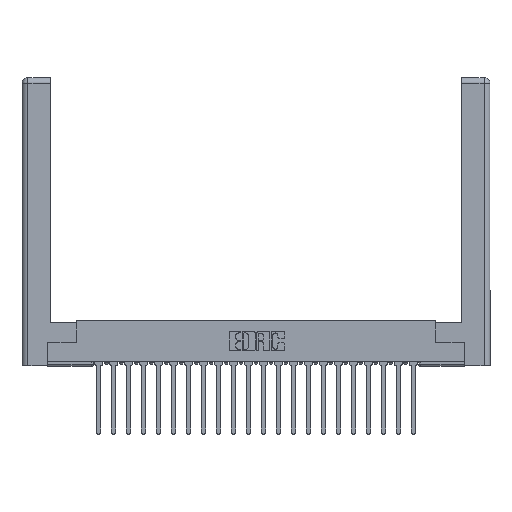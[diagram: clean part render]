
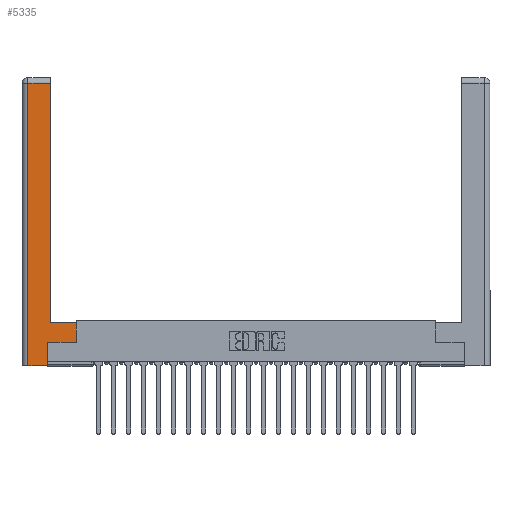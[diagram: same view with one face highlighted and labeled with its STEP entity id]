
A CAD part, top view. The second image highlights one B-rep face of the part: STEP entity #5335.
In plain terms, the highlighted planar face has unit normal (0, 0, 1).
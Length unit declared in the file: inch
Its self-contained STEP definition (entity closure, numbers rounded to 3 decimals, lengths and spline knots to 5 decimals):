
#131 = CARTESIAN_POINT ( 'NONE',  ( 0.0615, 2.94, 0. ) ) ;
#763 = VECTOR ( 'NONE', #1861, 39.37008 ) ;
#911 = EDGE_CURVE ( 'NONE', #6906, #17851, #3700, .T. ) ;
#1861 = DIRECTION ( 'NONE',  ( 0., 1., 0. ) ) ;
#2211 = DIRECTION ( 'NONE',  ( -1., 0., 0. ) ) ;
#2676 = VECTOR ( 'NONE', #22373, 39.37008 ) ;
#2912 = VECTOR ( 'NONE', #20176, 39.37008 ) ;
#2974 = LINE ( 'NONE', #18294, #2912 ) ;
#3685 = EDGE_CURVE ( 'NONE', #16562, #9395, #9204, .T. ) ;
#3700 = LINE ( 'NONE', #23017, #13595 ) ;
#4111 = LINE ( 'NONE', #131, #18956 ) ;
#4212 = FACE_OUTER_BOUND ( 'NONE', #11260, .T. ) ;
#4555 = LINE ( 'NONE', #8407, #15140 ) ;
#4575 = VERTEX_POINT ( 'NONE', #18118 ) ;
#4806 = CARTESIAN_POINT ( 'NONE',  ( 0.565, 0.45, 0. ) ) ;
#5335 = ADVANCED_FACE ( 'NONE', ( #4212 ), #17548, .F. ) ;
#5801 = DIRECTION ( 'NONE',  ( 0., 1., 0. ) ) ;
#5974 = EDGE_CURVE ( 'NONE', #4575, #16562, #4555, .T. ) ;
#6198 = CARTESIAN_POINT ( 'NONE',  ( 0., 0., 0. ) ) ;
#6542 = DIRECTION ( 'NONE',  ( 0., -1., 0. ) ) ;
#6906 = VERTEX_POINT ( 'NONE', #24538 ) ;
#7162 = ORIENTED_EDGE ( 'NONE', *, *, #12936, .T. ) ;
#7429 = LINE ( 'NONE', #13552, #24229 ) ;
#7552 = AXIS2_PLACEMENT_3D ( 'NONE', #6198, #19545, #23422 ) ;
#8185 = VERTEX_POINT ( 'NONE', #14827 ) ;
#8275 = VECTOR ( 'NONE', #14929, 39.37008 ) ;
#8407 = CARTESIAN_POINT ( 'NONE',  ( 0.0615, 0., 0. ) ) ;
#9204 = LINE ( 'NONE', #15975, #8275 ) ;
#9395 = VERTEX_POINT ( 'NONE', #11569 ) ;
#9710 = ORIENTED_EDGE ( 'NONE', *, *, #14147, .T. ) ;
#10265 = LINE ( 'NONE', #23746, #2676 ) ;
#11260 = EDGE_LOOP ( 'NONE', ( #15398, #7162, #13005, #13770, #14939, #9710, #16531, #13650 ) ) ;
#11569 = CARTESIAN_POINT ( 'NONE',  ( 0.265, 0., 0. ) ) ;
#12936 = EDGE_CURVE ( 'NONE', #8185, #4575, #4111, .T. ) ;
#13005 = ORIENTED_EDGE ( 'NONE', *, *, #5974, .T. ) ;
#13552 = CARTESIAN_POINT ( 'NONE',  ( 0.295, 0.45, 0. ) ) ;
#13595 = VECTOR ( 'NONE', #5801, 39.37008 ) ;
#13650 = ORIENTED_EDGE ( 'NONE', *, *, #23297, .T. ) ;
#13770 = ORIENTED_EDGE ( 'NONE', *, *, #3685, .T. ) ;
#14147 = EDGE_CURVE ( 'NONE', #21515, #6906, #10265, .T. ) ;
#14827 = CARTESIAN_POINT ( 'NONE',  ( 0.295, 2.94, 0. ) ) ;
#14929 = DIRECTION ( 'NONE',  ( 1., 0., 0. ) ) ;
#14936 = CARTESIAN_POINT ( 'NONE',  ( 0.0615, 0., 0. ) ) ;
#14939 = ORIENTED_EDGE ( 'NONE', *, *, #15290, .T. ) ;
#15050 = LINE ( 'NONE', #20807, #763 ) ;
#15140 = VECTOR ( 'NONE', #6542, 39.37008 ) ;
#15290 = EDGE_CURVE ( 'NONE', #9395, #21515, #15050, .T. ) ;
#15398 = ORIENTED_EDGE ( 'NONE', *, *, #20545, .T. ) ;
#15975 = CARTESIAN_POINT ( 'NONE',  ( 0.265, 0., 0. ) ) ;
#16531 = ORIENTED_EDGE ( 'NONE', *, *, #911, .T. ) ;
#16562 = VERTEX_POINT ( 'NONE', #14936 ) ;
#17548 = PLANE ( 'NONE',  #7552 ) ;
#17851 = VERTEX_POINT ( 'NONE', #4806 ) ;
#18118 = CARTESIAN_POINT ( 'NONE',  ( 0.0615, 2.94, 0. ) ) ;
#18294 = CARTESIAN_POINT ( 'NONE',  ( 0.295, 3., 0. ) ) ;
#18329 = CARTESIAN_POINT ( 'NONE',  ( 0.265, 0.245, 0. ) ) ;
#18637 = VERTEX_POINT ( 'NONE', #19205 ) ;
#18956 = VECTOR ( 'NONE', #19056, 39.37008 ) ;
#19056 = DIRECTION ( 'NONE',  ( -1., 0., 0. ) ) ;
#19205 = CARTESIAN_POINT ( 'NONE',  ( 0.295, 0.45, 0. ) ) ;
#19545 = DIRECTION ( 'NONE',  ( 0., 0., -1. ) ) ;
#20176 = DIRECTION ( 'NONE',  ( 0., 1., 0. ) ) ;
#20545 = EDGE_CURVE ( 'NONE', #18637, #8185, #2974, .T. ) ;
#20807 = CARTESIAN_POINT ( 'NONE',  ( 0.265, 0.245, 0. ) ) ;
#21515 = VERTEX_POINT ( 'NONE', #18329 ) ;
#22373 = DIRECTION ( 'NONE',  ( 1., 0., 0. ) ) ;
#23017 = CARTESIAN_POINT ( 'NONE',  ( 0.565, 0.45, 0. ) ) ;
#23297 = EDGE_CURVE ( 'NONE', #17851, #18637, #7429, .T. ) ;
#23422 = DIRECTION ( 'NONE',  ( -1., 0., 0. ) ) ;
#23746 = CARTESIAN_POINT ( 'NONE',  ( 0.565, 0.245, 0. ) ) ;
#24229 = VECTOR ( 'NONE', #2211, 39.37008 ) ;
#24538 = CARTESIAN_POINT ( 'NONE',  ( 0.565, 0.245, 0. ) ) ;
